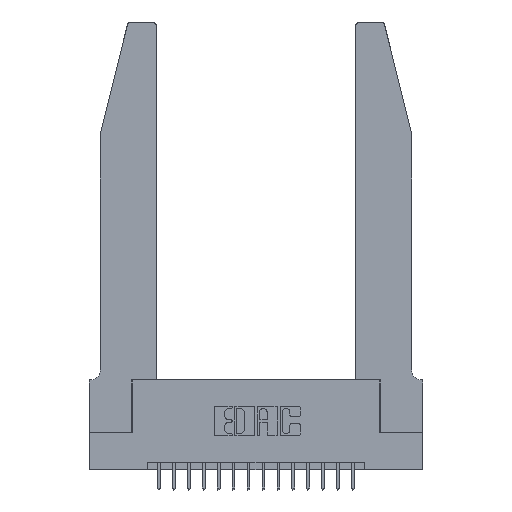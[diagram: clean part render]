
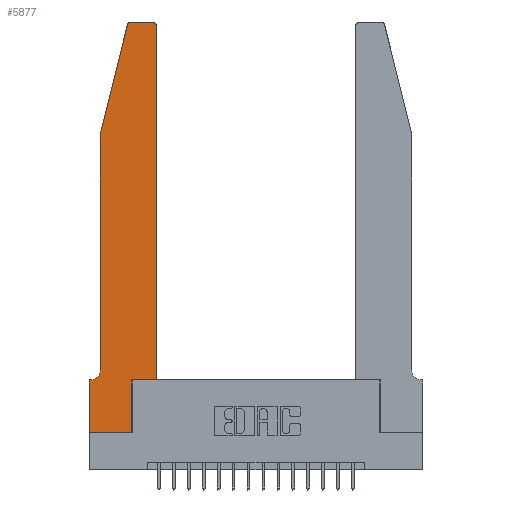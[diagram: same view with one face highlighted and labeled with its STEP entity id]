
A CAD part, top view. The second image highlights one B-rep face of the part: STEP entity #5877.
In plain terms, the highlighted planar face has unit normal (0, 0, 1).
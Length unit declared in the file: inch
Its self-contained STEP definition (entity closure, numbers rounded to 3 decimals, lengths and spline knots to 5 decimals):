
#242 = CARTESIAN_POINT ( 'NONE',  ( 0.4505, 2.72, 0.37 ) ) ;
#411 = DIRECTION ( 'NONE',  ( 0., 0., -1. ) ) ;
#855 = CARTESIAN_POINT ( 'NONE',  ( 0., 0., 0.37 ) ) ;
#923 = ORIENTED_EDGE ( 'NONE', *, *, #6663, .T. ) ;
#929 = DIRECTION ( 'NONE',  ( -1., 0., 0. ) ) ;
#1053 = VERTEX_POINT ( 'NONE', #10848 ) ;
#1104 = ORIENTED_EDGE ( 'NONE', *, *, #2795, .T. ) ;
#1151 = CARTESIAN_POINT ( 'NONE',  ( 0.2865, 0.35, 0.37 ) ) ;
#1331 = CARTESIAN_POINT ( 'NONE',  ( 0.2605, 2.75, 0.37 ) ) ;
#1958 = ORIENTED_EDGE ( 'NONE', *, *, #5434, .T. ) ;
#2795 = EDGE_CURVE ( 'NONE', #1053, #6451, #9178, .T. ) ;
#2970 = CARTESIAN_POINT ( 'NONE',  ( 0.4505, 0.35, 0.37 ) ) ;
#3264 = DIRECTION ( 'NONE',  ( 0., 0., 1. ) ) ;
#3376 = LINE ( 'NONE', #7746, #19486 ) ;
#3441 = VERTEX_POINT ( 'NONE', #8607 ) ;
#3535 = VERTEX_POINT ( 'NONE', #8003 ) ;
#3636 = DIRECTION ( 'NONE',  ( 0., 1., 0. ) ) ;
#3837 = CARTESIAN_POINT ( 'NONE',  ( 0.4505, 0.35, 0.37 ) ) ;
#4226 = DIRECTION ( 'NONE',  ( 0., 0., 1. ) ) ;
#4305 = CARTESIAN_POINT ( 'NONE',  ( 0.4505, 0.35, 0.37 ) ) ;
#4408 = DIRECTION ( 'NONE',  ( 0., 1., 0. ) ) ;
#5016 = LINE ( 'NONE', #3837, #19275 ) ;
#5205 = VERTEX_POINT ( 'NONE', #11625 ) ;
#5294 = VERTEX_POINT ( 'NONE', #1151 ) ;
#5434 = EDGE_CURVE ( 'NONE', #5205, #11660, #16430, .T. ) ;
#5607 = EDGE_CURVE ( 'NONE', #3535, #7440, #18707, .T. ) ;
#5712 = CARTESIAN_POINT ( 'NONE',  ( 0.284, 2.72, 0.37 ) ) ;
#5806 = VERTEX_POINT ( 'NONE', #2970 ) ;
#5811 = LINE ( 'NONE', #4305, #11152 ) ;
#5877 = ADVANCED_FACE ( 'NONE', ( #10602 ), #6257, .T. ) ;
#5949 = EDGE_CURVE ( 'NONE', #7440, #3441, #16874, .T. ) ;
#5958 = DIRECTION ( 'NONE',  ( 0., -1., 0. ) ) ;
#6257 = PLANE ( 'NONE',  #8604 ) ;
#6367 = DIRECTION ( 'NONE',  ( -0.239, -0.971, 0. ) ) ;
#6451 = VERTEX_POINT ( 'NONE', #17722 ) ;
#6663 = EDGE_CURVE ( 'NONE', #5294, #5806, #5811, .T. ) ;
#6720 = VECTOR ( 'NONE', #7381, 39.37008 ) ;
#6895 = DIRECTION ( 'NONE',  ( 1., 0., 0. ) ) ;
#7060 = CARTESIAN_POINT ( 'NONE',  ( 0.25487, 2.72718, 0.37 ) ) ;
#7153 = CARTESIAN_POINT ( 'NONE',  ( 0.4205, 2.72, 0.37 ) ) ;
#7198 = CIRCLE ( 'NONE', #13216, 0.03 ) ;
#7240 = DIRECTION ( 'NONE',  ( 1., 0., 0. ) ) ;
#7381 = DIRECTION ( 'NONE',  ( -1., 0., 0. ) ) ;
#7440 = VERTEX_POINT ( 'NONE', #15793 ) ;
#7746 = CARTESIAN_POINT ( 'NONE',  ( 0.0755, 2., 0.37 ) ) ;
#8003 = CARTESIAN_POINT ( 'NONE',  ( 0.0755, 2., 0.37 ) ) ;
#8541 = CARTESIAN_POINT ( 'NONE',  ( 0.0755, 2., 0.37 ) ) ;
#8604 = AXIS2_PLACEMENT_3D ( 'NONE', #12277, #3264, #9301 ) ;
#8607 = CARTESIAN_POINT ( 'NONE',  ( 0.0055, 0.35, 0.37 ) ) ;
#8633 = LINE ( 'NONE', #14500, #17996 ) ;
#9076 = ORIENTED_EDGE ( 'NONE', *, *, #13316, .T. ) ;
#9096 = DIRECTION ( 'NONE',  ( -1., 0., 0. ) ) ;
#9169 = EDGE_CURVE ( 'NONE', #14790, #5294, #18222, .T. ) ;
#9178 = LINE ( 'NONE', #19546, #15246 ) ;
#9188 = CARTESIAN_POINT ( 'NONE',  ( 0.2865, 0., 0.37 ) ) ;
#9236 = EDGE_CURVE ( 'NONE', #11660, #11314, #13455, .T. ) ;
#9301 = DIRECTION ( 'NONE',  ( 1., 0., 0. ) ) ;
#9390 = VERTEX_POINT ( 'NONE', #242 ) ;
#9446 = ORIENTED_EDGE ( 'NONE', *, *, #14191, .T. ) ;
#9548 = AXIS2_PLACEMENT_3D ( 'NONE', #16689, #411, #9096 ) ;
#9631 = EDGE_CURVE ( 'NONE', #6451, #14790, #14424, .T. ) ;
#10111 = DIRECTION ( 'NONE',  ( 0., 0., 1. ) ) ;
#10602 = FACE_OUTER_BOUND ( 'NONE', #15527, .T. ) ;
#10848 = CARTESIAN_POINT ( 'NONE',  ( 0., 0.35, 0.37 ) ) ;
#10991 = CARTESIAN_POINT ( 'NONE',  ( 0.284, 2.75, 0.37 ) ) ;
#11152 = VECTOR ( 'NONE', #19507, 39.37008 ) ;
#11314 = VERTEX_POINT ( 'NONE', #7060 ) ;
#11449 = ORIENTED_EDGE ( 'NONE', *, *, #5607, .T. ) ;
#11493 = ORIENTED_EDGE ( 'NONE', *, *, #9236, .T. ) ;
#11625 = CARTESIAN_POINT ( 'NONE',  ( 0.4205, 2.75, 0.37 ) ) ;
#11660 = VERTEX_POINT ( 'NONE', #10991 ) ;
#12277 = CARTESIAN_POINT ( 'NONE',  ( 0., 0.35, 0.37 ) ) ;
#13141 = AXIS2_PLACEMENT_3D ( 'NONE', #5712, #4226, #16345 ) ;
#13216 = AXIS2_PLACEMENT_3D ( 'NONE', #7153, #10111, #7240 ) ;
#13242 = CARTESIAN_POINT ( 'NONE',  ( 0.2865, 0.35, 0.37 ) ) ;
#13316 = EDGE_CURVE ( 'NONE', #11314, #3535, #3376, .T. ) ;
#13455 = CIRCLE ( 'NONE', #13141, 0.03 ) ;
#13662 = VECTOR ( 'NONE', #19097, 39.37008 ) ;
#13927 = ORIENTED_EDGE ( 'NONE', *, *, #16499, .T. ) ;
#14191 = EDGE_CURVE ( 'NONE', #5806, #9390, #5016, .T. ) ;
#14424 = LINE ( 'NONE', #855, #19512 ) ;
#14500 = CARTESIAN_POINT ( 'NONE',  ( 0.0755, 0.35, 0.37 ) ) ;
#14768 = ORIENTED_EDGE ( 'NONE', *, *, #9169, .T. ) ;
#14790 = VERTEX_POINT ( 'NONE', #9188 ) ;
#14946 = ORIENTED_EDGE ( 'NONE', *, *, #16614, .T. ) ;
#15190 = ORIENTED_EDGE ( 'NONE', *, *, #5949, .T. ) ;
#15246 = VECTOR ( 'NONE', #5958, 39.37008 ) ;
#15367 = VECTOR ( 'NONE', #4408, 39.37008 ) ;
#15527 = EDGE_LOOP ( 'NONE', ( #1958, #11493, #9076, #11449, #15190, #13927, #1104, #16651, #14768, #923, #9446, #14946 ) ) ;
#15793 = CARTESIAN_POINT ( 'NONE',  ( 0.0755, 0.42, 0.37 ) ) ;
#16345 = DIRECTION ( 'NONE',  ( 1., 0., 0. ) ) ;
#16430 = LINE ( 'NONE', #1331, #6720 ) ;
#16499 = EDGE_CURVE ( 'NONE', #3441, #1053, #8633, .T. ) ;
#16614 = EDGE_CURVE ( 'NONE', #9390, #5205, #7198, .T. ) ;
#16651 = ORIENTED_EDGE ( 'NONE', *, *, #9631, .T. ) ;
#16689 = CARTESIAN_POINT ( 'NONE',  ( 0.0055, 0.42, 0.37 ) ) ;
#16874 = CIRCLE ( 'NONE', #9548, 0.07 ) ;
#17722 = CARTESIAN_POINT ( 'NONE',  ( 0., 0., 0.37 ) ) ;
#17996 = VECTOR ( 'NONE', #929, 39.37008 ) ;
#18222 = LINE ( 'NONE', #13242, #15367 ) ;
#18707 = LINE ( 'NONE', #8541, #13662 ) ;
#19097 = DIRECTION ( 'NONE',  ( 0., -1., 0. ) ) ;
#19275 = VECTOR ( 'NONE', #3636, 39.37008 ) ;
#19486 = VECTOR ( 'NONE', #6367, 39.37008 ) ;
#19507 = DIRECTION ( 'NONE',  ( 1., 0., 0. ) ) ;
#19512 = VECTOR ( 'NONE', #6895, 39.37008 ) ;
#19546 = CARTESIAN_POINT ( 'NONE',  ( 0., 0., 0.37 ) ) ;
